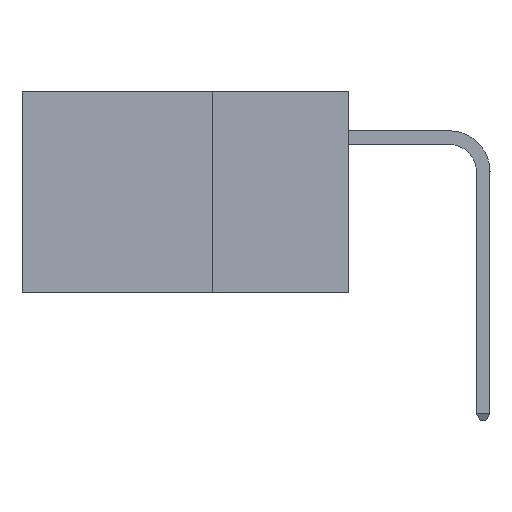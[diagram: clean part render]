
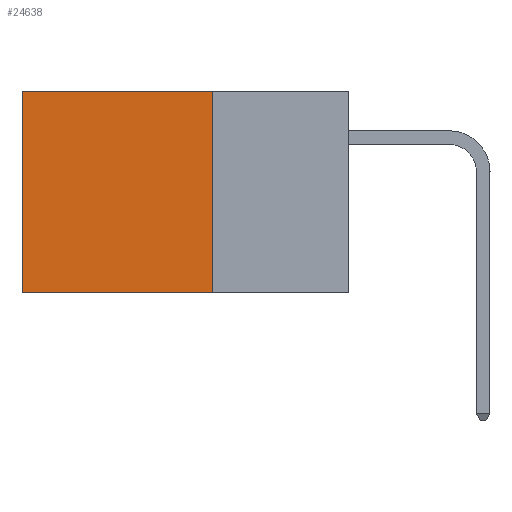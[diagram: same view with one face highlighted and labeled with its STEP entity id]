
A CAD part, left-side view. The second image highlights one B-rep face of the part: STEP entity #24638.
In plain terms, the highlighted planar face has unit normal (-1, 0, 0).
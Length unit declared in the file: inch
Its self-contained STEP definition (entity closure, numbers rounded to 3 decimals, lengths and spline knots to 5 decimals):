
#58 = CARTESIAN_POINT ( 'NONE',  ( 0.2875, 0.6, 0. ) ) ;
#842 = VERTEX_POINT ( 'NONE', #3304 ) ;
#1101 = LINE ( 'NONE', #3508, #30034 ) ;
#1544 = DIRECTION ( 'NONE',  ( 0., 0., -1. ) ) ;
#3304 = CARTESIAN_POINT ( 'NONE',  ( 0.2875, 0.6, 0. ) ) ;
#3508 = CARTESIAN_POINT ( 'NONE',  ( 0.2875, 0.25, 0. ) ) ;
#4787 = ORIENTED_EDGE ( 'NONE', *, *, #24469, .T. ) ;
#4962 = EDGE_CURVE ( 'NONE', #15109, #842, #14406, .T. ) ;
#5806 = DIRECTION ( 'NONE',  ( 0., 0., -1. ) ) ;
#6668 = VECTOR ( 'NONE', #5806, 39.37008 ) ;
#6978 = CARTESIAN_POINT ( 'NONE',  ( 0.2875, 0.6, -0.37 ) ) ;
#7063 = ORIENTED_EDGE ( 'NONE', *, *, #4962, .T. ) ;
#7359 = CARTESIAN_POINT ( 'NONE',  ( 0.2875, 0.25, 0. ) ) ;
#9256 = EDGE_LOOP ( 'NONE', ( #4787, #32845, #24519, #7063 ) ) ;
#9911 = VECTOR ( 'NONE', #29072, 39.37008 ) ;
#13518 = AXIS2_PLACEMENT_3D ( 'NONE', #18454, #18585, #1544 ) ;
#14406 = LINE ( 'NONE', #34572, #29958 ) ;
#14971 = DIRECTION ( 'NONE',  ( 0., 0., -1. ) ) ;
#15109 = VERTEX_POINT ( 'NONE', #7359 ) ;
#16590 = VERTEX_POINT ( 'NONE', #6978 ) ;
#18048 = DIRECTION ( 'NONE',  ( 0., 1., 0. ) ) ;
#18454 = CARTESIAN_POINT ( 'NONE',  ( 0.2875, 0.25, 0. ) ) ;
#18585 = DIRECTION ( 'NONE',  ( 1., 0., 0. ) ) ;
#19117 = VERTEX_POINT ( 'NONE', #25817 ) ;
#20558 = EDGE_CURVE ( 'NONE', #15109, #19117, #1101, .T. ) ;
#21692 = LINE ( 'NONE', #58, #6668 ) ;
#24469 = EDGE_CURVE ( 'NONE', #842, #16590, #21692, .T. ) ;
#24519 = ORIENTED_EDGE ( 'NONE', *, *, #20558, .F. ) ;
#24638 = ADVANCED_FACE ( 'NONE', ( #33042 ), #35110, .F. ) ;
#25817 = CARTESIAN_POINT ( 'NONE',  ( 0.2875, 0.25, -0.37 ) ) ;
#29072 = DIRECTION ( 'NONE',  ( 0., 1., 0. ) ) ;
#29958 = VECTOR ( 'NONE', #18048, 39.37008 ) ;
#30034 = VECTOR ( 'NONE', #14971, 39.37008 ) ;
#32066 = LINE ( 'NONE', #34591, #9911 ) ;
#32845 = ORIENTED_EDGE ( 'NONE', *, *, #35709, .F. ) ;
#33042 = FACE_OUTER_BOUND ( 'NONE', #9256, .T. ) ;
#34572 = CARTESIAN_POINT ( 'NONE',  ( 0.2875, 0.25, 0. ) ) ;
#34591 = CARTESIAN_POINT ( 'NONE',  ( 0.2875, 0.25, -0.37 ) ) ;
#35110 = PLANE ( 'NONE',  #13518 ) ;
#35709 = EDGE_CURVE ( 'NONE', #19117, #16590, #32066, .T. ) ;
